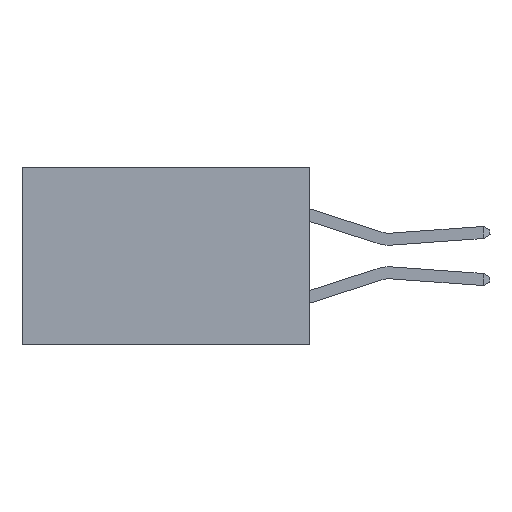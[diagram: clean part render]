
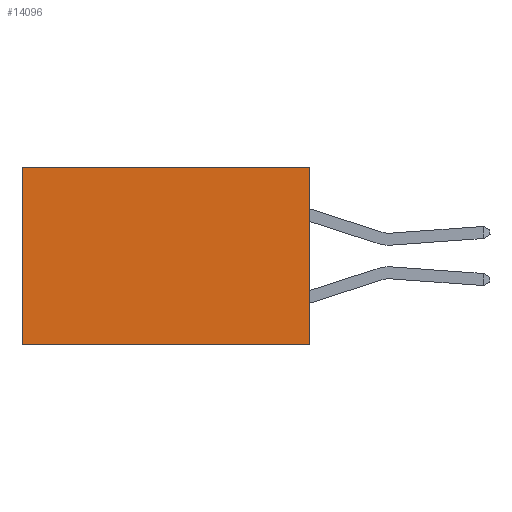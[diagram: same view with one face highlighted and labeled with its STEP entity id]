
A CAD part, left-side view. The second image highlights one B-rep face of the part: STEP entity #14096.
In plain terms, the highlighted planar face has unit normal (-1, 0, 0).
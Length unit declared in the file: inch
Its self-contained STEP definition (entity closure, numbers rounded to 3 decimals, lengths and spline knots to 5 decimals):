
#106 = EDGE_LOOP ( 'NONE', ( #11831, #9484, #10174, #10396 ) ) ;
#216 = VECTOR ( 'NONE', #3627, 39.37008 ) ;
#281 = CARTESIAN_POINT ( 'NONE',  ( 0.2615, 0., -0.37 ) ) ;
#743 = EDGE_CURVE ( 'NONE', #8411, #14138, #13391, .T. ) ;
#1015 = VERTEX_POINT ( 'NONE', #5757 ) ;
#1203 = CARTESIAN_POINT ( 'NONE',  ( 0.2615, 0.6, 0. ) ) ;
#1544 = DIRECTION ( 'NONE',  ( 0., 1., 0. ) ) ;
#2194 = VECTOR ( 'NONE', #14506, 39.37008 ) ;
#3430 = CARTESIAN_POINT ( 'NONE',  ( 0.2615, 0., 0. ) ) ;
#3627 = DIRECTION ( 'NONE',  ( 0., 0., -1. ) ) ;
#3682 = CARTESIAN_POINT ( 'NONE',  ( 0.2615, 0., 0. ) ) ;
#3925 = VECTOR ( 'NONE', #1544, 39.37008 ) ;
#5075 = DIRECTION ( 'NONE',  ( 0., 0., -1. ) ) ;
#5242 = EDGE_CURVE ( 'NONE', #1015, #14138, #7778, .T. ) ;
#5757 = CARTESIAN_POINT ( 'NONE',  ( 0.2615, 0., -0.37 ) ) ;
#5861 = LINE ( 'NONE', #14442, #216 ) ;
#6243 = CARTESIAN_POINT ( 'NONE',  ( 0.2615, 0.6, -0.37 ) ) ;
#6668 = CARTESIAN_POINT ( 'NONE',  ( 0.2615, 0., -0.37 ) ) ;
#7009 = AXIS2_PLACEMENT_3D ( 'NONE', #281, #7539, #5075 ) ;
#7459 = FACE_OUTER_BOUND ( 'NONE', #106, .T. ) ;
#7537 = VECTOR ( 'NONE', #9278, 39.37008 ) ;
#7539 = DIRECTION ( 'NONE',  ( 1., 0., 0. ) ) ;
#7778 = LINE ( 'NONE', #6668, #3925 ) ;
#7831 = LINE ( 'NONE', #3430, #7537 ) ;
#8411 = VERTEX_POINT ( 'NONE', #1203 ) ;
#9145 = VERTEX_POINT ( 'NONE', #3682 ) ;
#9278 = DIRECTION ( 'NONE',  ( 0., 1., 0. ) ) ;
#9484 = ORIENTED_EDGE ( 'NONE', *, *, #5242, .F. ) ;
#10174 = ORIENTED_EDGE ( 'NONE', *, *, #14268, .F. ) ;
#10396 = ORIENTED_EDGE ( 'NONE', *, *, #14609, .T. ) ;
#11693 = CARTESIAN_POINT ( 'NONE',  ( 0.2615, 0.6, -0.37 ) ) ;
#11831 = ORIENTED_EDGE ( 'NONE', *, *, #743, .T. ) ;
#12236 = PLANE ( 'NONE',  #7009 ) ;
#13391 = LINE ( 'NONE', #6243, #2194 ) ;
#14096 = ADVANCED_FACE ( 'NONE', ( #7459 ), #12236, .F. ) ;
#14138 = VERTEX_POINT ( 'NONE', #11693 ) ;
#14268 = EDGE_CURVE ( 'NONE', #9145, #1015, #5861, .T. ) ;
#14442 = CARTESIAN_POINT ( 'NONE',  ( 0.2615, 0., -0.37 ) ) ;
#14506 = DIRECTION ( 'NONE',  ( 0., 0., -1. ) ) ;
#14609 = EDGE_CURVE ( 'NONE', #9145, #8411, #7831, .T. ) ;
